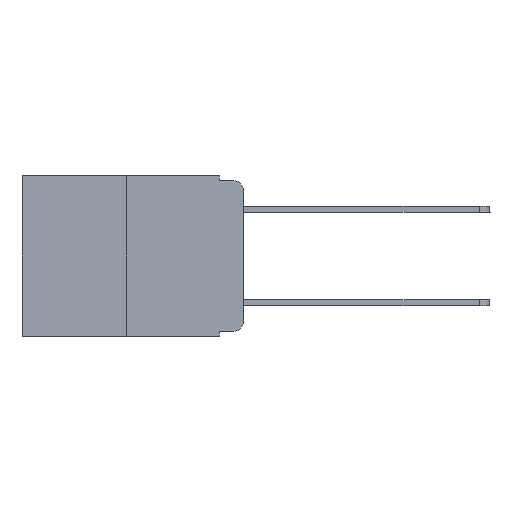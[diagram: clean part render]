
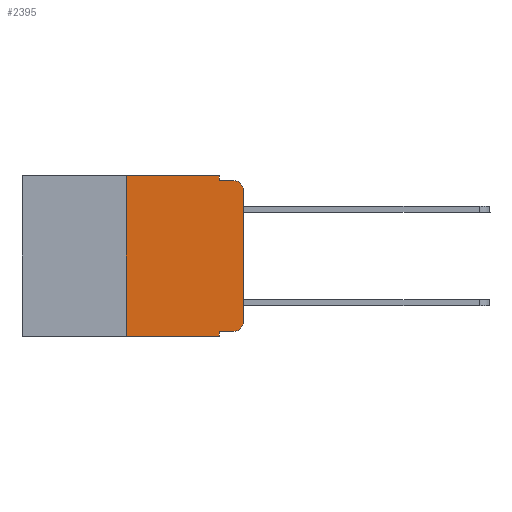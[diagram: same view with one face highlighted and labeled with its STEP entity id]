
A CAD part, left-side view. The second image highlights one B-rep face of the part: STEP entity #2395.
In plain terms, the highlighted planar face has unit normal (-1, 0, 0).
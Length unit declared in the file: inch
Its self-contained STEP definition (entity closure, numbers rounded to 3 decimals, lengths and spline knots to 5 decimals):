
#47 = FACE_OUTER_BOUND ( 'NONE', #10174, .T. ) ;
#187 = CARTESIAN_POINT ( 'NONE',  ( 0., 0.02, -0.333 ) ) ;
#912 = EDGE_CURVE ( 'NONE', #6981, #20983, #2617, .T. ) ;
#1075 = EDGE_CURVE ( 'NONE', #8969, #4076, #4923, .T. ) ;
#1274 = ORIENTED_EDGE ( 'NONE', *, *, #912, .F. ) ;
#1433 = PLANE ( 'NONE',  #9377 ) ;
#1463 = ORIENTED_EDGE ( 'NONE', *, *, #21790, .T. ) ;
#1624 = CARTESIAN_POINT ( 'NONE',  ( 0., 0., -0.313 ) ) ;
#1981 = DIRECTION ( 'NONE',  ( -1., 0., 0. ) ) ;
#2255 = DIRECTION ( 'NONE',  ( 0., 0., 1. ) ) ;
#2395 = ADVANCED_FACE ( 'NONE', ( #47 ), #1433, .F. ) ;
#2591 = VECTOR ( 'NONE', #16894, 39.37008 ) ;
#2617 = LINE ( 'NONE', #22676, #15259 ) ;
#2620 = ORIENTED_EDGE ( 'NONE', *, *, #13661, .T. ) ;
#2658 = VERTEX_POINT ( 'NONE', #21550 ) ;
#2761 = DIRECTION ( 'NONE',  ( 0., -1., 0. ) ) ;
#2777 = CARTESIAN_POINT ( 'NONE',  ( 0., 0.25, 0. ) ) ;
#3161 = CARTESIAN_POINT ( 'NONE',  ( 0., 0.25, -0.343 ) ) ;
#3209 = VECTOR ( 'NONE', #2761, 39.37008 ) ;
#3238 = DIRECTION ( 'NONE',  ( 0., -1., 0. ) ) ;
#3894 = EDGE_CURVE ( 'NONE', #18518, #18728, #13483, .T. ) ;
#3929 = ORIENTED_EDGE ( 'NONE', *, *, #3894, .T. ) ;
#4076 = VERTEX_POINT ( 'NONE', #20991 ) ;
#4125 = EDGE_CURVE ( 'NONE', #20983, #7634, #8394, .T. ) ;
#4530 = VERTEX_POINT ( 'NONE', #16818 ) ;
#4548 = ORIENTED_EDGE ( 'NONE', *, *, #10878, .F. ) ;
#4635 = EDGE_CURVE ( 'NONE', #8969, #2658, #10886, .T. ) ;
#4923 = LINE ( 'NONE', #2777, #2591 ) ;
#5067 = VECTOR ( 'NONE', #22373, 39.37008 ) ;
#5099 = DIRECTION ( 'NONE',  ( 0., 0., -1. ) ) ;
#5103 = CIRCLE ( 'NONE', #15782, 0.02 ) ;
#6981 = VERTEX_POINT ( 'NONE', #21335 ) ;
#7542 = CARTESIAN_POINT ( 'NONE',  ( 0., 0.02, -0.313 ) ) ;
#7634 = VERTEX_POINT ( 'NONE', #10649 ) ;
#7770 = ORIENTED_EDGE ( 'NONE', *, *, #1075, .F. ) ;
#8082 = CARTESIAN_POINT ( 'NONE',  ( 0., 0.051, -0.333 ) ) ;
#8374 = EDGE_CURVE ( 'NONE', #18728, #7634, #5103, .T. ) ;
#8394 = LINE ( 'NONE', #20840, #14018 ) ;
#8969 = VERTEX_POINT ( 'NONE', #3161 ) ;
#9377 = AXIS2_PLACEMENT_3D ( 'NONE', #19299, #23128, #10452 ) ;
#10004 = ORIENTED_EDGE ( 'NONE', *, *, #8374, .T. ) ;
#10174 = EDGE_LOOP ( 'NONE', ( #3929, #10004, #11523, #1274, #20932, #7770, #13498, #4548, #1463, #2620 ) ) ;
#10452 = DIRECTION ( 'NONE',  ( 0., 0., -1. ) ) ;
#10649 = CARTESIAN_POINT ( 'NONE',  ( 0., 0.02, -0.01 ) ) ;
#10878 = EDGE_CURVE ( 'NONE', #4530, #2658, #23138, .T. ) ;
#10886 = LINE ( 'NONE', #13388, #5067 ) ;
#11523 = ORIENTED_EDGE ( 'NONE', *, *, #4125, .F. ) ;
#11601 = VECTOR ( 'NONE', #16872, 39.37008 ) ;
#12124 = DIRECTION ( 'NONE',  ( 0., 0., -1. ) ) ;
#12312 = CARTESIAN_POINT ( 'NONE',  ( 0., 0.02, -0.03 ) ) ;
#13270 = CARTESIAN_POINT ( 'NONE',  ( 0., 0.473, 0. ) ) ;
#13302 = CARTESIAN_POINT ( 'NONE',  ( 0., 0., -0.03 ) ) ;
#13388 = CARTESIAN_POINT ( 'NONE',  ( 0., 0.473, -0.343 ) ) ;
#13483 = LINE ( 'NONE', #22153, #16539 ) ;
#13498 = ORIENTED_EDGE ( 'NONE', *, *, #4635, .T. ) ;
#13661 = EDGE_CURVE ( 'NONE', #14282, #18518, #23003, .T. ) ;
#13887 = DIRECTION ( 'NONE',  ( 0., 0., -1. ) ) ;
#14018 = VECTOR ( 'NONE', #3238, 39.37008 ) ;
#14113 = DIRECTION ( 'NONE',  ( -1., 0., 0. ) ) ;
#14183 = VECTOR ( 'NONE', #5099, 39.37008 ) ;
#14282 = VERTEX_POINT ( 'NONE', #187 ) ;
#14489 = CARTESIAN_POINT ( 'NONE',  ( 0., 0.051, -0.01 ) ) ;
#15259 = VECTOR ( 'NONE', #12124, 39.37008 ) ;
#15782 = AXIS2_PLACEMENT_3D ( 'NONE', #12312, #14113, #13887 ) ;
#16539 = VECTOR ( 'NONE', #2255, 39.37008 ) ;
#16818 = CARTESIAN_POINT ( 'NONE',  ( 0., 0.051, -0.333 ) ) ;
#16872 = DIRECTION ( 'NONE',  ( 0., -1., 0. ) ) ;
#16894 = DIRECTION ( 'NONE',  ( 0., 0., 1. ) ) ;
#18232 = AXIS2_PLACEMENT_3D ( 'NONE', #7542, #1981, #21804 ) ;
#18518 = VERTEX_POINT ( 'NONE', #1624 ) ;
#18728 = VERTEX_POINT ( 'NONE', #13302 ) ;
#18879 = LINE ( 'NONE', #8082, #3209 ) ;
#19299 = CARTESIAN_POINT ( 'NONE',  ( 0., 0.473, 0. ) ) ;
#20840 = CARTESIAN_POINT ( 'NONE',  ( 0., 0.051, -0.01 ) ) ;
#20932 = ORIENTED_EDGE ( 'NONE', *, *, #21826, .F. ) ;
#20983 = VERTEX_POINT ( 'NONE', #14489 ) ;
#20991 = CARTESIAN_POINT ( 'NONE',  ( 0., 0.25, 0. ) ) ;
#21335 = CARTESIAN_POINT ( 'NONE',  ( 0., 0.051, 0. ) ) ;
#21550 = CARTESIAN_POINT ( 'NONE',  ( 0., 0.051, -0.343 ) ) ;
#21790 = EDGE_CURVE ( 'NONE', #4530, #14282, #18879, .T. ) ;
#21804 = DIRECTION ( 'NONE',  ( 0., 0., -1. ) ) ;
#21826 = EDGE_CURVE ( 'NONE', #4076, #6981, #22221, .T. ) ;
#22153 = CARTESIAN_POINT ( 'NONE',  ( 0., 0., 0. ) ) ;
#22221 = LINE ( 'NONE', #13270, #11601 ) ;
#22373 = DIRECTION ( 'NONE',  ( 0., -1., 0. ) ) ;
#22676 = CARTESIAN_POINT ( 'NONE',  ( 0., 0.051, 0. ) ) ;
#22896 = CARTESIAN_POINT ( 'NONE',  ( 0., 0.051, 0. ) ) ;
#23003 = CIRCLE ( 'NONE', #18232, 0.02 ) ;
#23128 = DIRECTION ( 'NONE',  ( 1., 0., 0. ) ) ;
#23138 = LINE ( 'NONE', #22896, #14183 ) ;
